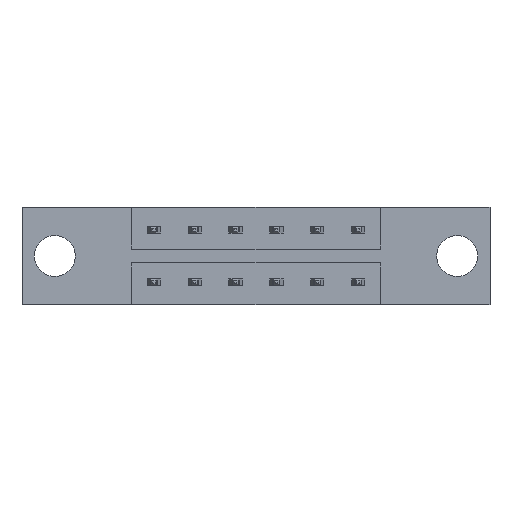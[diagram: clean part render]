
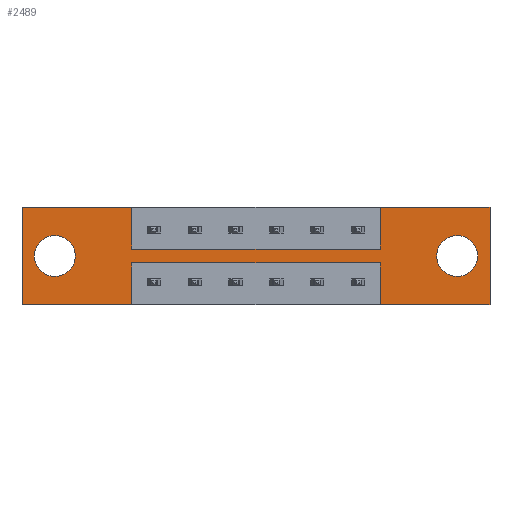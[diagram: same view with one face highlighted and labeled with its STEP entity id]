
A CAD part, front view. The second image highlights one B-rep face of the part: STEP entity #2489.
In plain terms, the highlighted planar face has unit normal (0, -1, 0).
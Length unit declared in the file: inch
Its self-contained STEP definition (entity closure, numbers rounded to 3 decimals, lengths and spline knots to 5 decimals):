
#4 = CARTESIAN_POINT ( 'NONE',  ( 0.125, 0., -0.185 ) ) ;
#9 = CARTESIAN_POINT ( 'NONE',  ( 0., 0., -0.37 ) ) ;
#140 = FACE_OUTER_BOUND ( 'NONE', #6947, .T. ) ;
#208 = PLANE ( 'NONE',  #7464 ) ;
#317 = DIRECTION ( 'NONE',  ( 0., 1., 0. ) ) ;
#352 = CIRCLE ( 'NONE', #4968, 0.078 ) ;
#381 = AXIS2_PLACEMENT_3D ( 'NONE', #688, #546, #6835 ) ;
#396 = ORIENTED_EDGE ( 'NONE', *, *, #4134, .F. ) ;
#543 = CIRCLE ( 'NONE', #1299, 0.078 ) ;
#546 = DIRECTION ( 'NONE',  ( 0., 1., 0. ) ) ;
#574 = VECTOR ( 'NONE', #5958, 39.37008 ) ;
#581 = EDGE_LOOP ( 'NONE', ( #6982, #8238 ) ) ;
#621 = VERTEX_POINT ( 'NONE', #6578 ) ;
#688 = CARTESIAN_POINT ( 'NONE',  ( 1.659, 0., -0.185 ) ) ;
#781 = CARTESIAN_POINT ( 'NONE',  ( 1.3665, 0., -0.37 ) ) ;
#825 = ORIENTED_EDGE ( 'NONE', *, *, #6955, .F. ) ;
#845 = LINE ( 'NONE', #6355, #4361 ) ;
#870 = LINE ( 'NONE', #4480, #7734 ) ;
#896 = VERTEX_POINT ( 'NONE', #4780 ) ;
#930 = CARTESIAN_POINT ( 'NONE',  ( 0.4175, 0., -0.2115 ) ) ;
#958 = CARTESIAN_POINT ( 'NONE',  ( 0.4175, 0., -0.1585 ) ) ;
#978 = LINE ( 'NONE', #958, #4488 ) ;
#1139 = VECTOR ( 'NONE', #6950, 39.37008 ) ;
#1180 = DIRECTION ( 'NONE',  ( 1., 0., 0. ) ) ;
#1239 = VECTOR ( 'NONE', #1878, 39.37008 ) ;
#1299 = AXIS2_PLACEMENT_3D ( 'NONE', #4497, #317, #5155 ) ;
#1473 = VERTEX_POINT ( 'NONE', #4159 ) ;
#1480 = VECTOR ( 'NONE', #7217, 39.37008 ) ;
#1507 = VERTEX_POINT ( 'NONE', #2144 ) ;
#1668 = DIRECTION ( 'NONE',  ( 0., 0., 1. ) ) ;
#1700 = VERTEX_POINT ( 'NONE', #5538 ) ;
#1728 = ORIENTED_EDGE ( 'NONE', *, *, #2308, .T. ) ;
#1878 = DIRECTION ( 'NONE',  ( 1., 0., 0. ) ) ;
#1938 = EDGE_CURVE ( 'NONE', #7600, #621, #7292, .T. ) ;
#1944 = ORIENTED_EDGE ( 'NONE', *, *, #8544, .F. ) ;
#2119 = LINE ( 'NONE', #7211, #7282 ) ;
#2144 = CARTESIAN_POINT ( 'NONE',  ( 0.125, 0., -0.263 ) ) ;
#2263 = VERTEX_POINT ( 'NONE', #781 ) ;
#2308 = EDGE_CURVE ( 'NONE', #6075, #1507, #4606, .T. ) ;
#2406 = CARTESIAN_POINT ( 'NONE',  ( 0.4175, 0., 0. ) ) ;
#2449 = ORIENTED_EDGE ( 'NONE', *, *, #7532, .F. ) ;
#2456 = CARTESIAN_POINT ( 'NONE',  ( 0.125, 0., -0.185 ) ) ;
#2489 = ADVANCED_FACE ( 'NONE', ( #5406, #8502, #140 ), #208, .T. ) ;
#2693 = ORIENTED_EDGE ( 'NONE', *, *, #3902, .F. ) ;
#2781 = VERTEX_POINT ( 'NONE', #3474 ) ;
#2801 = CARTESIAN_POINT ( 'NONE',  ( 1.784, 0., 0. ) ) ;
#3079 = LINE ( 'NONE', #6325, #1139 ) ;
#3171 = CARTESIAN_POINT ( 'NONE',  ( 0., 0., 0. ) ) ;
#3238 = DIRECTION ( 'NONE',  ( 0., -1., 0. ) ) ;
#3445 = VECTOR ( 'NONE', #6453, 39.37008 ) ;
#3474 = CARTESIAN_POINT ( 'NONE',  ( 1.784, 0., -0.37 ) ) ;
#3587 = CARTESIAN_POINT ( 'NONE',  ( 0.4175, 0., -0.37 ) ) ;
#3707 = VECTOR ( 'NONE', #8220, 39.37008 ) ;
#3785 = CARTESIAN_POINT ( 'NONE',  ( 1.659, 0., -0.263 ) ) ;
#3863 = DIRECTION ( 'NONE',  ( 0., 0., 1. ) ) ;
#3902 = EDGE_CURVE ( 'NONE', #1473, #5967, #7665, .T. ) ;
#3935 = ORIENTED_EDGE ( 'NONE', *, *, #5027, .F. ) ;
#3968 = DIRECTION ( 'NONE',  ( 0., 0., -1. ) ) ;
#4031 = CARTESIAN_POINT ( 'NONE',  ( 1.3665, 0., -0.1585 ) ) ;
#4085 = VERTEX_POINT ( 'NONE', #4547 ) ;
#4114 = DIRECTION ( 'NONE',  ( 0., 0., -1. ) ) ;
#4134 = EDGE_CURVE ( 'NONE', #6856, #4085, #7934, .T. ) ;
#4144 = ORIENTED_EDGE ( 'NONE', *, *, #5494, .F. ) ;
#4159 = CARTESIAN_POINT ( 'NONE',  ( 1.3665, 0., -0.2115 ) ) ;
#4233 = VERTEX_POINT ( 'NONE', #3171 ) ;
#4294 = VERTEX_POINT ( 'NONE', #2406 ) ;
#4342 = ORIENTED_EDGE ( 'NONE', *, *, #6877, .F. ) ;
#4361 = VECTOR ( 'NONE', #6981, 39.37008 ) ;
#4389 = DIRECTION ( 'NONE',  ( 0., 1., 0. ) ) ;
#4397 = VECTOR ( 'NONE', #3863, 39.37008 ) ;
#4472 = CARTESIAN_POINT ( 'NONE',  ( 0., 0., -0.37 ) ) ;
#4480 = CARTESIAN_POINT ( 'NONE',  ( 0.4175, 0., -0.1585 ) ) ;
#4482 = EDGE_CURVE ( 'NONE', #1507, #6075, #352, .T. ) ;
#4488 = VECTOR ( 'NONE', #1180, 39.37008 ) ;
#4497 = CARTESIAN_POINT ( 'NONE',  ( 1.659, 0., -0.185 ) ) ;
#4520 = EDGE_CURVE ( 'NONE', #2263, #1473, #5638, .T. ) ;
#4547 = CARTESIAN_POINT ( 'NONE',  ( 1.3665, 0., 0. ) ) ;
#4599 = EDGE_CURVE ( 'NONE', #4233, #4294, #5024, .T. ) ;
#4606 = CIRCLE ( 'NONE', #8302, 0.078 ) ;
#4780 = CARTESIAN_POINT ( 'NONE',  ( 0., 0., -0.37 ) ) ;
#4968 = AXIS2_PLACEMENT_3D ( 'NONE', #4, #8532, #8396 ) ;
#5024 = LINE ( 'NONE', #6741, #1480 ) ;
#5027 = EDGE_CURVE ( 'NONE', #8162, #2781, #2119, .T. ) ;
#5046 = CARTESIAN_POINT ( 'NONE',  ( 0.4175, 0., -0.2115 ) ) ;
#5155 = DIRECTION ( 'NONE',  ( 0., 0., -1. ) ) ;
#5224 = EDGE_CURVE ( 'NONE', #4294, #1700, #870, .T. ) ;
#5386 = CARTESIAN_POINT ( 'NONE',  ( 0., 0., 0. ) ) ;
#5406 = FACE_BOUND ( 'NONE', #581, .T. ) ;
#5467 = ORIENTED_EDGE ( 'NONE', *, *, #4482, .T. ) ;
#5494 = EDGE_CURVE ( 'NONE', #1700, #6856, #978, .T. ) ;
#5538 = CARTESIAN_POINT ( 'NONE',  ( 0.4175, 0., -0.1585 ) ) ;
#5638 = LINE ( 'NONE', #8033, #3707 ) ;
#5689 = ORIENTED_EDGE ( 'NONE', *, *, #8004, .F. ) ;
#5877 = ORIENTED_EDGE ( 'NONE', *, *, #5224, .F. ) ;
#5958 = DIRECTION ( 'NONE',  ( -1., 0., 0. ) ) ;
#5967 = VERTEX_POINT ( 'NONE', #5046 ) ;
#6016 = CARTESIAN_POINT ( 'NONE',  ( 0.4175, 0., -0.2115 ) ) ;
#6075 = VERTEX_POINT ( 'NONE', #7613 ) ;
#6121 = EDGE_CURVE ( 'NONE', #621, #7600, #543, .T. ) ;
#6325 = CARTESIAN_POINT ( 'NONE',  ( 0., 0., 0. ) ) ;
#6355 = CARTESIAN_POINT ( 'NONE',  ( 0., 0., -0.37 ) ) ;
#6390 = DIRECTION ( 'NONE',  ( 0., 0., -1. ) ) ;
#6453 = DIRECTION ( 'NONE',  ( -1., 0., 0. ) ) ;
#6578 = CARTESIAN_POINT ( 'NONE',  ( 1.659, 0., -0.107 ) ) ;
#6683 = VERTEX_POINT ( 'NONE', #3587 ) ;
#6741 = CARTESIAN_POINT ( 'NONE',  ( 0., 0., 0. ) ) ;
#6835 = DIRECTION ( 'NONE',  ( 0., 0., -1. ) ) ;
#6856 = VERTEX_POINT ( 'NONE', #8122 ) ;
#6873 = EDGE_LOOP ( 'NONE', ( #1728, #5467 ) ) ;
#6877 = EDGE_CURVE ( 'NONE', #6683, #896, #845, .T. ) ;
#6947 = EDGE_LOOP ( 'NONE', ( #7149, #1944, #3935, #5689, #396, #4144, #5877, #7526, #2449, #4342, #825, #2693 ) ) ;
#6950 = DIRECTION ( 'NONE',  ( 0., 0., 1. ) ) ;
#6955 = EDGE_CURVE ( 'NONE', #5967, #6683, #7710, .T. ) ;
#6961 = DIRECTION ( 'NONE',  ( 0., 0., -1. ) ) ;
#6981 = DIRECTION ( 'NONE',  ( -1., 0., 0. ) ) ;
#6982 = ORIENTED_EDGE ( 'NONE', *, *, #6121, .T. ) ;
#7149 = ORIENTED_EDGE ( 'NONE', *, *, #4520, .F. ) ;
#7165 = VECTOR ( 'NONE', #6390, 39.37008 ) ;
#7211 = CARTESIAN_POINT ( 'NONE',  ( 1.784, 0., 0. ) ) ;
#7217 = DIRECTION ( 'NONE',  ( 1., 0., 0. ) ) ;
#7282 = VECTOR ( 'NONE', #6961, 39.37008 ) ;
#7292 = CIRCLE ( 'NONE', #381, 0.078 ) ;
#7464 = AXIS2_PLACEMENT_3D ( 'NONE', #9, #3238, #3968 ) ;
#7526 = ORIENTED_EDGE ( 'NONE', *, *, #4599, .F. ) ;
#7532 = EDGE_CURVE ( 'NONE', #896, #4233, #3079, .T. ) ;
#7600 = VERTEX_POINT ( 'NONE', #3785 ) ;
#7613 = CARTESIAN_POINT ( 'NONE',  ( 0.125, 0., -0.107 ) ) ;
#7665 = LINE ( 'NONE', #6016, #574 ) ;
#7710 = LINE ( 'NONE', #930, #7165 ) ;
#7734 = VECTOR ( 'NONE', #4114, 39.37008 ) ;
#7934 = LINE ( 'NONE', #4031, #4397 ) ;
#8004 = EDGE_CURVE ( 'NONE', #4085, #8162, #8170, .T. ) ;
#8033 = CARTESIAN_POINT ( 'NONE',  ( 1.3665, 0., -0.2115 ) ) ;
#8122 = CARTESIAN_POINT ( 'NONE',  ( 1.3665, 0., -0.1585 ) ) ;
#8162 = VERTEX_POINT ( 'NONE', #2801 ) ;
#8170 = LINE ( 'NONE', #5386, #1239 ) ;
#8220 = DIRECTION ( 'NONE',  ( 0., 0., 1. ) ) ;
#8238 = ORIENTED_EDGE ( 'NONE', *, *, #1938, .T. ) ;
#8302 = AXIS2_PLACEMENT_3D ( 'NONE', #2456, #4389, #1668 ) ;
#8396 = DIRECTION ( 'NONE',  ( 0., 0., 1. ) ) ;
#8476 = LINE ( 'NONE', #4472, #3445 ) ;
#8502 = FACE_BOUND ( 'NONE', #6873, .T. ) ;
#8532 = DIRECTION ( 'NONE',  ( 0., 1., 0. ) ) ;
#8544 = EDGE_CURVE ( 'NONE', #2781, #2263, #8476, .T. ) ;
